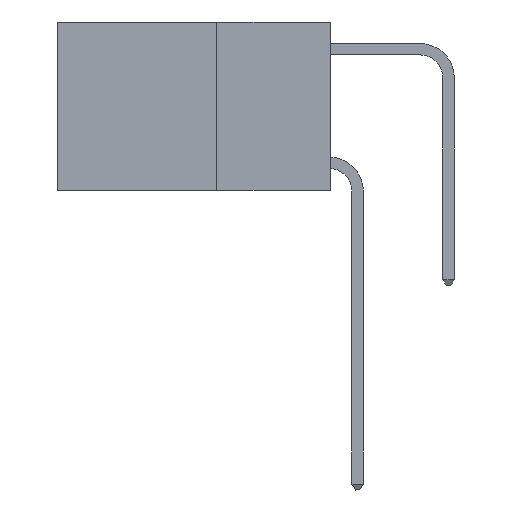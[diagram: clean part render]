
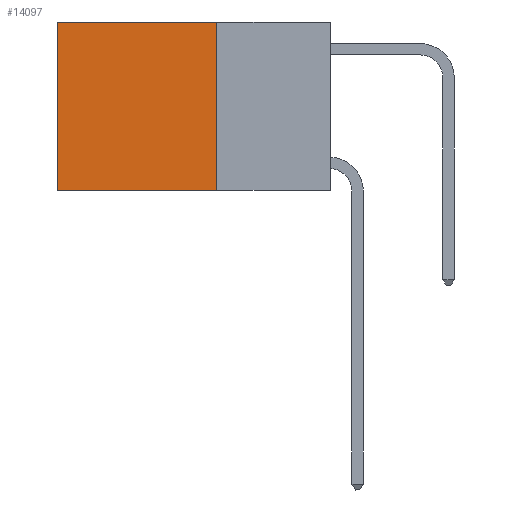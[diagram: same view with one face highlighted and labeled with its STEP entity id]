
A CAD part, left-side view. The second image highlights one B-rep face of the part: STEP entity #14097.
In plain terms, the highlighted planar face has unit normal (-1, 0, 0).
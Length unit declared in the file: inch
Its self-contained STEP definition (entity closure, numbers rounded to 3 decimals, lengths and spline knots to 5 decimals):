
#322 = EDGE_CURVE ( 'NONE', #12055, #2905, #16948, .T. ) ;
#1336 = ORIENTED_EDGE ( 'NONE', *, *, #12562, .F. ) ;
#2073 = DIRECTION ( 'NONE',  ( 0., 0., -1. ) ) ;
#2665 = CARTESIAN_POINT ( 'NONE',  ( 0.2625, 0.25, 0. ) ) ;
#2783 = CARTESIAN_POINT ( 'NONE',  ( 0.2625, 0.25, -0.37 ) ) ;
#2905 = VERTEX_POINT ( 'NONE', #7936 ) ;
#3007 = VECTOR ( 'NONE', #9608, 39.37008 ) ;
#3759 = DIRECTION ( 'NONE',  ( 0., 0., -1. ) ) ;
#3765 = EDGE_CURVE ( 'NONE', #8317, #13777, #9529, .T. ) ;
#4545 = EDGE_CURVE ( 'NONE', #2905, #13777, #10874, .T. ) ;
#5627 = VECTOR ( 'NONE', #8139, 39.37008 ) ;
#6429 = DIRECTION ( 'NONE',  ( 0., 0., -1. ) ) ;
#7148 = ORIENTED_EDGE ( 'NONE', *, *, #322, .T. ) ;
#7186 = CARTESIAN_POINT ( 'NONE',  ( 0.2625, 0.6, -0.37 ) ) ;
#7824 = EDGE_LOOP ( 'NONE', ( #13081, #9743, #1336, #7148 ) ) ;
#7936 = CARTESIAN_POINT ( 'NONE',  ( 0.2625, 0.6, 0. ) ) ;
#8139 = DIRECTION ( 'NONE',  ( 0., 1., 0. ) ) ;
#8317 = VERTEX_POINT ( 'NONE', #2783 ) ;
#8920 = CARTESIAN_POINT ( 'NONE',  ( 0.2625, 0.25, 0. ) ) ;
#8933 = VECTOR ( 'NONE', #3759, 39.37008 ) ;
#9529 = LINE ( 'NONE', #11981, #5627 ) ;
#9608 = DIRECTION ( 'NONE',  ( 0., 1., 0. ) ) ;
#9743 = ORIENTED_EDGE ( 'NONE', *, *, #3765, .F. ) ;
#10076 = CARTESIAN_POINT ( 'NONE',  ( 0.2625, 0.25, 0. ) ) ;
#10783 = DIRECTION ( 'NONE',  ( 1., 0., 0. ) ) ;
#10874 = LINE ( 'NONE', #13685, #8933 ) ;
#11907 = AXIS2_PLACEMENT_3D ( 'NONE', #13502, #10783, #6429 ) ;
#11981 = CARTESIAN_POINT ( 'NONE',  ( 0.2625, 0.25, -0.37 ) ) ;
#12055 = VERTEX_POINT ( 'NONE', #10076 ) ;
#12562 = EDGE_CURVE ( 'NONE', #12055, #8317, #14804, .T. ) ;
#13081 = ORIENTED_EDGE ( 'NONE', *, *, #4545, .T. ) ;
#13502 = CARTESIAN_POINT ( 'NONE',  ( 0.2625, 0.25, 0. ) ) ;
#13685 = CARTESIAN_POINT ( 'NONE',  ( 0.2625, 0.6, 0. ) ) ;
#13777 = VERTEX_POINT ( 'NONE', #7186 ) ;
#13947 = VECTOR ( 'NONE', #2073, 39.37008 ) ;
#14097 = ADVANCED_FACE ( 'NONE', ( #16750 ), #16395, .F. ) ;
#14804 = LINE ( 'NONE', #8920, #13947 ) ;
#16395 = PLANE ( 'NONE',  #11907 ) ;
#16750 = FACE_OUTER_BOUND ( 'NONE', #7824, .T. ) ;
#16948 = LINE ( 'NONE', #2665, #3007 ) ;
